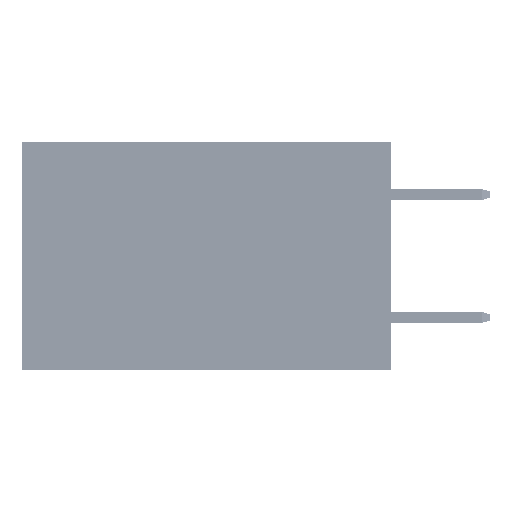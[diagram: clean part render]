
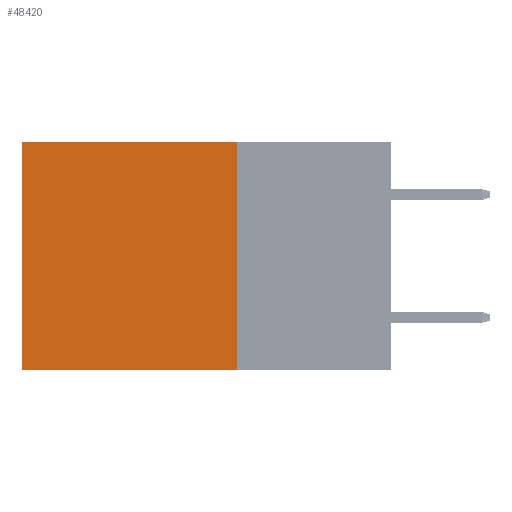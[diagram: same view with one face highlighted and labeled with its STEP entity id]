
A CAD part, left-side view. The second image highlights one B-rep face of the part: STEP entity #48420.
In plain terms, the highlighted planar face has unit normal (-1, 0, 0).
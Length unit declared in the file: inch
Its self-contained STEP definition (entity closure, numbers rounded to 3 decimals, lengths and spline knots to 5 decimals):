
#2957 = VERTEX_POINT ( 'NONE', #20430 ) ;
#3242 = DIRECTION ( 'NONE',  ( 1., 0., 0. ) ) ;
#4730 = EDGE_CURVE ( 'NONE', #2957, #41138, #31457, .T. ) ;
#5615 = VECTOR ( 'NONE', #15496, 39.37008 ) ;
#5846 = CARTESIAN_POINT ( 'NONE',  ( 0.2875, 0.25, 0. ) ) ;
#7742 = EDGE_CURVE ( 'NONE', #44995, #21483, #27202, .T. ) ;
#9492 = ORIENTED_EDGE ( 'NONE', *, *, #25697, .F. ) ;
#12993 = ORIENTED_EDGE ( 'NONE', *, *, #7742, .F. ) ;
#14509 = VECTOR ( 'NONE', #36199, 39.37008 ) ;
#15496 = DIRECTION ( 'NONE',  ( 0., 0., -1. ) ) ;
#15700 = VECTOR ( 'NONE', #39899, 39.37008 ) ;
#16778 = EDGE_CURVE ( 'NONE', #44995, #2957, #36238, .T. ) ;
#18495 = DIRECTION ( 'NONE',  ( 0., 0., -1. ) ) ;
#19452 = CARTESIAN_POINT ( 'NONE',  ( 0.2875, 0.25, -0.37 ) ) ;
#20430 = CARTESIAN_POINT ( 'NONE',  ( 0.2875, 0.6, 0. ) ) ;
#21161 = PLANE ( 'NONE',  #41922 ) ;
#21483 = VERTEX_POINT ( 'NONE', #19452 ) ;
#25697 = EDGE_CURVE ( 'NONE', #21483, #41138, #32137, .T. ) ;
#27202 = LINE ( 'NONE', #36924, #30726 ) ;
#28478 = ORIENTED_EDGE ( 'NONE', *, *, #4730, .T. ) ;
#29584 = DIRECTION ( 'NONE',  ( 0., 0., -1. ) ) ;
#30726 = VECTOR ( 'NONE', #29584, 39.37008 ) ;
#31457 = LINE ( 'NONE', #34194, #5615 ) ;
#32137 = LINE ( 'NONE', #42386, #15700 ) ;
#32479 = CARTESIAN_POINT ( 'NONE',  ( 0.2875, 0.25, 0. ) ) ;
#32725 = FACE_OUTER_BOUND ( 'NONE', #43870, .T. ) ;
#33006 = ORIENTED_EDGE ( 'NONE', *, *, #16778, .T. ) ;
#34194 = CARTESIAN_POINT ( 'NONE',  ( 0.2875, 0.6, 0. ) ) ;
#36199 = DIRECTION ( 'NONE',  ( 0., 1., 0. ) ) ;
#36238 = LINE ( 'NONE', #5846, #14509 ) ;
#36471 = CARTESIAN_POINT ( 'NONE',  ( 0.2875, 0.6, -0.37 ) ) ;
#36924 = CARTESIAN_POINT ( 'NONE',  ( 0.2875, 0.25, 0. ) ) ;
#39899 = DIRECTION ( 'NONE',  ( 0., 1., 0. ) ) ;
#41138 = VERTEX_POINT ( 'NONE', #36471 ) ;
#41922 = AXIS2_PLACEMENT_3D ( 'NONE', #32479, #3242, #18495 ) ;
#42386 = CARTESIAN_POINT ( 'NONE',  ( 0.2875, 0.25, -0.37 ) ) ;
#43516 = CARTESIAN_POINT ( 'NONE',  ( 0.2875, 0.25, 0. ) ) ;
#43870 = EDGE_LOOP ( 'NONE', ( #28478, #9492, #12993, #33006 ) ) ;
#44995 = VERTEX_POINT ( 'NONE', #43516 ) ;
#48420 = ADVANCED_FACE ( 'NONE', ( #32725 ), #21161, .F. ) ;
